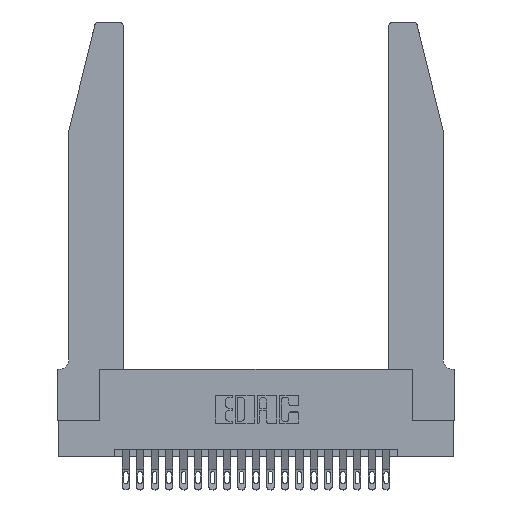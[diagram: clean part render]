
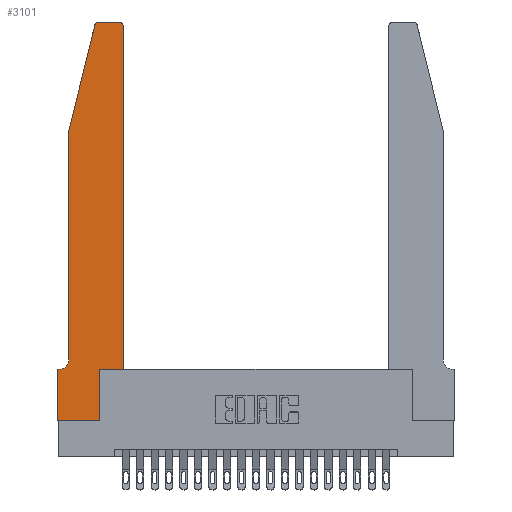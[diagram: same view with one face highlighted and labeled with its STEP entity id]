
A CAD part, top view. The second image highlights one B-rep face of the part: STEP entity #3101.
In plain terms, the highlighted planar face has unit normal (0, 0, 1).
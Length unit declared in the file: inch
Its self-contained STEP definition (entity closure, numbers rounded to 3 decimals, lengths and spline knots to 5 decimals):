
#133 = CARTESIAN_POINT ( 'NONE',  ( 0.0055, 0.35, 0.37 ) ) ;
#169 = EDGE_CURVE ( 'NONE', #19518, #8168, #14144, .T. ) ;
#184 = VERTEX_POINT ( 'NONE', #18956 ) ;
#423 = CIRCLE ( 'NONE', #12981, 0.03 ) ;
#580 = VERTEX_POINT ( 'NONE', #8591 ) ;
#711 = VECTOR ( 'NONE', #12062, 39.37008 ) ;
#1643 = LINE ( 'NONE', #12592, #4133 ) ;
#1666 = ORIENTED_EDGE ( 'NONE', *, *, #169, .T. ) ;
#2163 = CARTESIAN_POINT ( 'NONE',  ( 0.4505, 0.35, 0.37 ) ) ;
#2460 = EDGE_CURVE ( 'NONE', #8737, #580, #17917, .T. ) ;
#3101 = ADVANCED_FACE ( 'NONE', ( #16527 ), #21050, .T. ) ;
#3437 = VECTOR ( 'NONE', #10615, 39.37008 ) ;
#4133 = VECTOR ( 'NONE', #19724, 39.37008 ) ;
#4157 = CARTESIAN_POINT ( 'NONE',  ( 0.0055, 0.42, 0.37 ) ) ;
#4238 = VERTEX_POINT ( 'NONE', #18164 ) ;
#4451 = VECTOR ( 'NONE', #7496, 39.37008 ) ;
#4587 = DIRECTION ( 'NONE',  ( -1., 0., 0. ) ) ;
#4713 = VERTEX_POINT ( 'NONE', #14119 ) ;
#4816 = VECTOR ( 'NONE', #9705, 39.37008 ) ;
#4990 = EDGE_CURVE ( 'NONE', #4238, #22251, #18937, .T. ) ;
#5002 = ORIENTED_EDGE ( 'NONE', *, *, #10513, .T. ) ;
#5043 = CARTESIAN_POINT ( 'NONE',  ( 0.284, 2.75, 0.37 ) ) ;
#5137 = CARTESIAN_POINT ( 'NONE',  ( 0.284, 2.72, 0.37 ) ) ;
#5912 = LINE ( 'NONE', #8047, #4816 ) ;
#5993 = CARTESIAN_POINT ( 'NONE',  ( 0.4205, 2.72, 0.37 ) ) ;
#6015 = ORIENTED_EDGE ( 'NONE', *, *, #18580, .T. ) ;
#6174 = AXIS2_PLACEMENT_3D ( 'NONE', #5137, #13868, #6899 ) ;
#6899 = DIRECTION ( 'NONE',  ( 1., 0., 0. ) ) ;
#7028 = LINE ( 'NONE', #9809, #7311 ) ;
#7031 = ORIENTED_EDGE ( 'NONE', *, *, #11330, .T. ) ;
#7311 = VECTOR ( 'NONE', #7987, 39.37008 ) ;
#7496 = DIRECTION ( 'NONE',  ( 1., 0., 0. ) ) ;
#7724 = CARTESIAN_POINT ( 'NONE',  ( 0.0755, 0.42, 0.37 ) ) ;
#7987 = DIRECTION ( 'NONE',  ( -1., 0., 0. ) ) ;
#8047 = CARTESIAN_POINT ( 'NONE',  ( 0.0755, 2., 0.37 ) ) ;
#8168 = VERTEX_POINT ( 'NONE', #5043 ) ;
#8485 = CARTESIAN_POINT ( 'NONE',  ( 0.4505, 0.35, 0.37 ) ) ;
#8591 = CARTESIAN_POINT ( 'NONE',  ( 0.2865, 0.35, 0.37 ) ) ;
#8737 = VERTEX_POINT ( 'NONE', #12776 ) ;
#8803 = DIRECTION ( 'NONE',  ( 1., 0., 0. ) ) ;
#8809 = VERTEX_POINT ( 'NONE', #7724 ) ;
#9334 = CIRCLE ( 'NONE', #14338, 0.07 ) ;
#9690 = VECTOR ( 'NONE', #4587, 39.37008 ) ;
#9705 = DIRECTION ( 'NONE',  ( 0., -1., 0. ) ) ;
#9809 = CARTESIAN_POINT ( 'NONE',  ( 0.0755, 0.35, 0.37 ) ) ;
#9935 = EDGE_CURVE ( 'NONE', #4713, #19518, #423, .T. ) ;
#10390 = DIRECTION ( 'NONE',  ( 0., 0., 1. ) ) ;
#10402 = AXIS2_PLACEMENT_3D ( 'NONE', #17653, #10390, #22848 ) ;
#10513 = EDGE_CURVE ( 'NONE', #8809, #22207, #9334, .T. ) ;
#10615 = DIRECTION ( 'NONE',  ( 1., 0., 0. ) ) ;
#10795 = ORIENTED_EDGE ( 'NONE', *, *, #2460, .T. ) ;
#11330 = EDGE_CURVE ( 'NONE', #22207, #16799, #7028, .T. ) ;
#11603 = EDGE_CURVE ( 'NONE', #184, #8737, #22964, .T. ) ;
#11739 = VECTOR ( 'NONE', #18210, 39.37008 ) ;
#11959 = EDGE_CURVE ( 'NONE', #22251, #8809, #5912, .T. ) ;
#12062 = DIRECTION ( 'NONE',  ( 0., 1., 0. ) ) ;
#12279 = ORIENTED_EDGE ( 'NONE', *, *, #11959, .T. ) ;
#12403 = VECTOR ( 'NONE', #22638, 39.37008 ) ;
#12592 = CARTESIAN_POINT ( 'NONE',  ( 0., 0., 0.37 ) ) ;
#12776 = CARTESIAN_POINT ( 'NONE',  ( 0.2865, 0., 0.37 ) ) ;
#12981 = AXIS2_PLACEMENT_3D ( 'NONE', #5993, #22761, #8803 ) ;
#12982 = CARTESIAN_POINT ( 'NONE',  ( 0.0755, 2., 0.37 ) ) ;
#13659 = ORIENTED_EDGE ( 'NONE', *, *, #4990, .T. ) ;
#13868 = DIRECTION ( 'NONE',  ( 0., 0., 1. ) ) ;
#14119 = CARTESIAN_POINT ( 'NONE',  ( 0.4505, 2.72, 0.37 ) ) ;
#14144 = LINE ( 'NONE', #15396, #9690 ) ;
#14188 = ORIENTED_EDGE ( 'NONE', *, *, #11603, .T. ) ;
#14338 = AXIS2_PLACEMENT_3D ( 'NONE', #4157, #18363, #20668 ) ;
#14566 = CARTESIAN_POINT ( 'NONE',  ( 0., 0.35, 0.37 ) ) ;
#14645 = CARTESIAN_POINT ( 'NONE',  ( 0.0755, 2., 0.37 ) ) ;
#15081 = EDGE_LOOP ( 'NONE', ( #1666, #15868, #13659, #12279, #5002, #7031, #6015, #14188, #10795, #19672, #20782, #17720 ) ) ;
#15373 = CARTESIAN_POINT ( 'NONE',  ( 0.2865, 0.35, 0.37 ) ) ;
#15396 = CARTESIAN_POINT ( 'NONE',  ( 0.2605, 2.75, 0.37 ) ) ;
#15754 = EDGE_CURVE ( 'NONE', #8168, #4238, #15996, .T. ) ;
#15868 = ORIENTED_EDGE ( 'NONE', *, *, #15754, .T. ) ;
#15996 = CIRCLE ( 'NONE', #6174, 0.03 ) ;
#16527 = FACE_OUTER_BOUND ( 'NONE', #15081, .T. ) ;
#16799 = VERTEX_POINT ( 'NONE', #14566 ) ;
#16836 = LINE ( 'NONE', #8485, #711 ) ;
#17513 = LINE ( 'NONE', #17947, #4451 ) ;
#17653 = CARTESIAN_POINT ( 'NONE',  ( 0., 0.35, 0.37 ) ) ;
#17720 = ORIENTED_EDGE ( 'NONE', *, *, #9935, .T. ) ;
#17917 = LINE ( 'NONE', #15373, #12403 ) ;
#17947 = CARTESIAN_POINT ( 'NONE',  ( 0.4505, 0.35, 0.37 ) ) ;
#18061 = EDGE_CURVE ( 'NONE', #580, #20446, #17513, .T. ) ;
#18164 = CARTESIAN_POINT ( 'NONE',  ( 0.25487, 2.72718, 0.37 ) ) ;
#18210 = DIRECTION ( 'NONE',  ( -0.239, -0.971, 0. ) ) ;
#18363 = DIRECTION ( 'NONE',  ( 0., 0., -1. ) ) ;
#18580 = EDGE_CURVE ( 'NONE', #16799, #184, #1643, .T. ) ;
#18937 = LINE ( 'NONE', #14645, #11739 ) ;
#18956 = CARTESIAN_POINT ( 'NONE',  ( 0., 0., 0.37 ) ) ;
#19518 = VERTEX_POINT ( 'NONE', #22336 ) ;
#19672 = ORIENTED_EDGE ( 'NONE', *, *, #18061, .T. ) ;
#19724 = DIRECTION ( 'NONE',  ( 0., -1., 0. ) ) ;
#20446 = VERTEX_POINT ( 'NONE', #2163 ) ;
#20668 = DIRECTION ( 'NONE',  ( -1., 0., 0. ) ) ;
#20782 = ORIENTED_EDGE ( 'NONE', *, *, #21877, .T. ) ;
#21050 = PLANE ( 'NONE',  #10402 ) ;
#21877 = EDGE_CURVE ( 'NONE', #20446, #4713, #16836, .T. ) ;
#22207 = VERTEX_POINT ( 'NONE', #133 ) ;
#22251 = VERTEX_POINT ( 'NONE', #12982 ) ;
#22336 = CARTESIAN_POINT ( 'NONE',  ( 0.4205, 2.75, 0.37 ) ) ;
#22638 = DIRECTION ( 'NONE',  ( 0., 1., 0. ) ) ;
#22761 = DIRECTION ( 'NONE',  ( 0., 0., 1. ) ) ;
#22835 = CARTESIAN_POINT ( 'NONE',  ( 0., 0., 0.37 ) ) ;
#22848 = DIRECTION ( 'NONE',  ( 1., 0., 0. ) ) ;
#22964 = LINE ( 'NONE', #22835, #3437 ) ;
